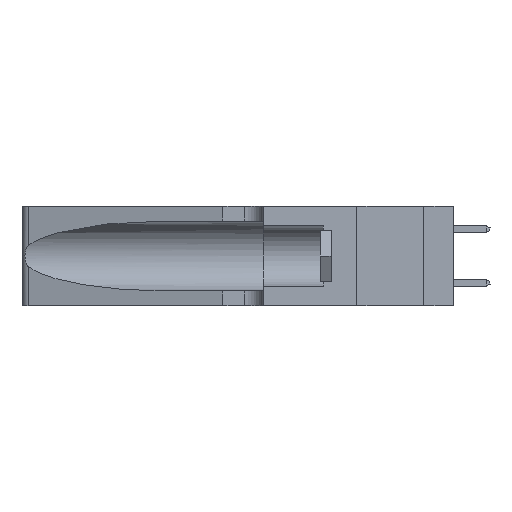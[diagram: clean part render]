
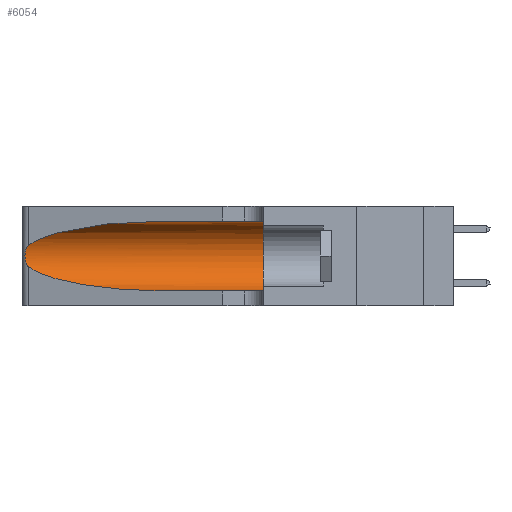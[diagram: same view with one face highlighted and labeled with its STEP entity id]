
A CAD part, left-side view. The second image highlights one B-rep face of the part: STEP entity #6054.
In plain terms, the highlighted cylindrical face has radius 3.308 mm (diameter 6.617 mm), a partial arc.
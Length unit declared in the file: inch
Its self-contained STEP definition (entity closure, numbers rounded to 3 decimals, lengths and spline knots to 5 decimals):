
#403 = ORIENTED_EDGE ( 'NONE', *, *, #3505, .T. ) ;
#506 = CARTESIAN_POINT ( 'NONE',  ( 0.2373, 1.15595, 0.28018 ) ) ;
#735 = DIRECTION ( 'NONE',  ( 0., -1., 0. ) ) ;
#1044 = B_SPLINE_CURVE_WITH_KNOTS ( 'NONE', 3,
 ( #21105, #13922, #14008, #3050, #15785, #4915, #17600, #6795, #19394, #8619, #21189, #10467, #22994, #12292 ),
 .UNSPECIFIED., .F., .F.,
 ( 4, 2, 2, 2, 2, 2, 4 ),
 ( 0., 0.00027, 0.00053, 0.00107, 0.0016, 0.00187, 0.00214 ),
 .UNSPECIFIED. ) ;
#2122 =( BOUNDED_CURVE ( )  B_SPLINE_CURVE ( 3, ( #3321, #21378, #23174, #16061 ),
 .UNSPECIFIED., .F., .T. ) 
 B_SPLINE_CURVE_WITH_KNOTS ( ( 4, 4 ),
 ( 3.44316, 4.71239 ),
 .UNSPECIFIED. ) 
 CURVE ( )  GEOMETRIC_REPRESENTATION_ITEM ( )  RATIONAL_B_SPLINE_CURVE ( ( 1., 0.87, 0.87, 1. ) ) 
 REPRESENTATION_ITEM ( '' )  );
#2343 = CARTESIAN_POINT ( 'NONE',  ( 0.1305, 0.72297, 0.31525 ) ) ;
#2641 = CARTESIAN_POINT ( 'NONE',  ( 0.1305, 1.61858, 0.05475 ) ) ;
#3050 = CARTESIAN_POINT ( 'NONE',  ( 0.25787, 1.23484, 0.2124 ) ) ;
#3321 = CARTESIAN_POINT ( 'NONE',  ( 0.25487, 1.22718, 0.14631 ) ) ;
#3505 = EDGE_CURVE ( 'NONE', #13172, #20987, #2122, .T. ) ;
#4158 = ORIENTED_EDGE ( 'NONE', *, *, #8078, .T. ) ;
#4491 = DIRECTION ( 'NONE',  ( 0., -1., 0. ) ) ;
#4915 = CARTESIAN_POINT ( 'NONE',  ( 0.26018, 1.23835, 0.19895 ) ) ;
#5008 = CARTESIAN_POINT ( 'NONE',  ( 0.1305, 0.35, 0.31525 ) ) ;
#5063 = ORIENTED_EDGE ( 'NONE', *, *, #7520, .F. ) ;
#5635 = VECTOR ( 'NONE', #735, 39.37008 ) ;
#6054 = ADVANCED_FACE ( 'NONE', ( #8540 ), #11689, .F. ) ;
#6243 = LINE ( 'NONE', #22558, #5635 ) ;
#6477 = EDGE_LOOP ( 'NONE', ( #19954, #14879, #403, #4158, #23039, #5063 ) ) ;
#6558 = CARTESIAN_POINT ( 'NONE',  ( 0.1305, 0.35, 0.05475 ) ) ;
#6654 = DIRECTION ( 'NONE',  ( 0., 0., -1. ) ) ;
#6697 = DIRECTION ( 'NONE',  ( 0., 1., 0. ) ) ;
#6795 = CARTESIAN_POINT ( 'NONE',  ( 0.26075, 1.23896, 0.178 ) ) ;
#6896 = CARTESIAN_POINT ( 'NONE',  ( 0.25487, 1.22718, 0.22369 ) ) ;
#7520 = EDGE_CURVE ( 'NONE', #14638, #16470, #6243, .T. ) ;
#8078 = EDGE_CURVE ( 'NONE', #20987, #8136, #22569, .T. ) ;
#8136 = VERTEX_POINT ( 'NONE', #6558 ) ;
#8331 = AXIS2_PLACEMENT_3D ( 'NONE', #22852, #12069, #6654 ) ;
#8540 = FACE_OUTER_BOUND ( 'NONE', #6477, .T. ) ;
#8619 = CARTESIAN_POINT ( 'NONE',  ( 0.25856, 1.23593, 0.16098 ) ) ;
#10467 = CARTESIAN_POINT ( 'NONE',  ( 0.25639, 1.23186, 0.15144 ) ) ;
#11000 = EDGE_CURVE ( 'NONE', #12355, #13172, #1044, .T. ) ;
#11112 = CARTESIAN_POINT ( 'NONE',  ( 0.1305, 0.72297, 0.31525 ) ) ;
#11261 = CIRCLE ( 'NONE', #12092, 0.13025 ) ;
#11689 = CYLINDRICAL_SURFACE ( 'NONE', #8331, 0.13025 ) ;
#12069 = DIRECTION ( 'NONE',  ( 0., -1., 0. ) ) ;
#12092 = AXIS2_PLACEMENT_3D ( 'NONE', #17503, #6697, #19298 ) ;
#12292 = CARTESIAN_POINT ( 'NONE',  ( 0.25487, 1.22718, 0.14631 ) ) ;
#12355 = VERTEX_POINT ( 'NONE', #6896 ) ;
#13040 = VECTOR ( 'NONE', #4491, 39.37008 ) ;
#13172 = VERTEX_POINT ( 'NONE', #13990 ) ;
#13413 = CARTESIAN_POINT ( 'NONE',  ( 0.25487, 1.22718, 0.22369 ) ) ;
#13922 = CARTESIAN_POINT ( 'NONE',  ( 0.25555, 1.22994, 0.2215 ) ) ;
#13990 = CARTESIAN_POINT ( 'NONE',  ( 0.25487, 1.22718, 0.14631 ) ) ;
#14008 = CARTESIAN_POINT ( 'NONE',  ( 0.25639, 1.23184, 0.21858 ) ) ;
#14638 = VERTEX_POINT ( 'NONE', #11112 ) ;
#14879 = ORIENTED_EDGE ( 'NONE', *, *, #11000, .T. ) ;
#15785 = CARTESIAN_POINT ( 'NONE',  ( 0.25854, 1.2359, 0.20912 ) ) ;
#16028 =( BOUNDED_CURVE ( )  B_SPLINE_CURVE ( 3, ( #2343, #18665, #506, #13413 ),
 .UNSPECIFIED., .F., .F. ) 
 B_SPLINE_CURVE_WITH_KNOTS ( ( 4, 4 ),
 ( 1.5708, 2.84003 ),
 .UNSPECIFIED. ) 
 CURVE ( )  GEOMETRIC_REPRESENTATION_ITEM ( )  RATIONAL_B_SPLINE_CURVE ( ( 1., 0.87, 0.87, 1. ) ) 
 REPRESENTATION_ITEM ( '' )  );
#16061 = CARTESIAN_POINT ( 'NONE',  ( 0.1305, 0.72297, 0.05475 ) ) ;
#16470 = VERTEX_POINT ( 'NONE', #5008 ) ;
#17503 = CARTESIAN_POINT ( 'NONE',  ( 0.1305, 0.35, 0.185 ) ) ;
#17600 = CARTESIAN_POINT ( 'NONE',  ( 0.26075, 1.23896, 0.19203 ) ) ;
#18665 = CARTESIAN_POINT ( 'NONE',  ( 0.18966, 0.96281, 0.31525 ) ) ;
#18944 = EDGE_CURVE ( 'NONE', #16470, #8136, #11261, .T. ) ;
#19298 = DIRECTION ( 'NONE',  ( 0., 0., 1. ) ) ;
#19394 = CARTESIAN_POINT ( 'NONE',  ( 0.26017, 1.23833, 0.17102 ) ) ;
#19954 = ORIENTED_EDGE ( 'NONE', *, *, #23492, .T. ) ;
#20987 = VERTEX_POINT ( 'NONE', #21310 ) ;
#21105 = CARTESIAN_POINT ( 'NONE',  ( 0.25487, 1.22718, 0.22369 ) ) ;
#21189 = CARTESIAN_POINT ( 'NONE',  ( 0.25789, 1.23486, 0.15765 ) ) ;
#21310 = CARTESIAN_POINT ( 'NONE',  ( 0.1305, 0.72297, 0.05475 ) ) ;
#21378 = CARTESIAN_POINT ( 'NONE',  ( 0.2373, 1.15595, 0.08982 ) ) ;
#22558 = CARTESIAN_POINT ( 'NONE',  ( 0.1305, 1.61858, 0.31525 ) ) ;
#22569 = LINE ( 'NONE', #2641, #13040 ) ;
#22852 = CARTESIAN_POINT ( 'NONE',  ( 0.1305, 1.61858, 0.185 ) ) ;
#22994 = CARTESIAN_POINT ( 'NONE',  ( 0.25555, 1.22993, 0.14849 ) ) ;
#23039 = ORIENTED_EDGE ( 'NONE', *, *, #18944, .F. ) ;
#23174 = CARTESIAN_POINT ( 'NONE',  ( 0.18966, 0.96281, 0.05475 ) ) ;
#23492 = EDGE_CURVE ( 'NONE', #14638, #12355, #16028, .T. ) ;
